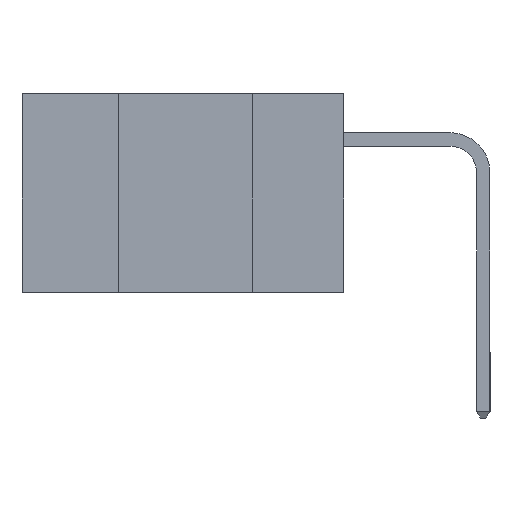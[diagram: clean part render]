
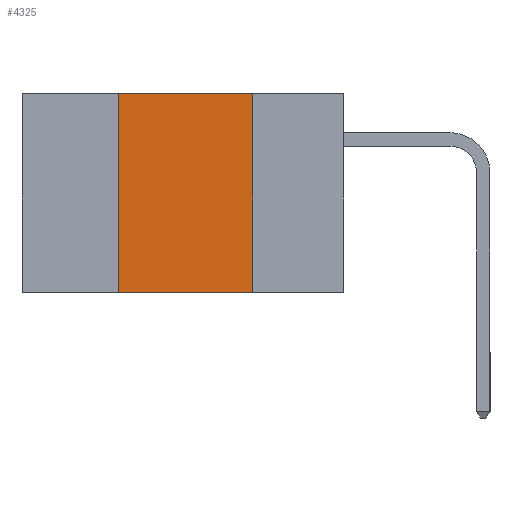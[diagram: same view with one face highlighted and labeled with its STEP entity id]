
A CAD part, left-side view. The second image highlights one B-rep face of the part: STEP entity #4325.
In plain terms, the highlighted planar face has unit normal (-1, 0, 0).
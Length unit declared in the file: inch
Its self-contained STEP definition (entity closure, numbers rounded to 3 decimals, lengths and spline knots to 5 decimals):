
#7 = VERTEX_POINT ( 'NONE', #14242 ) ;
#102 = CARTESIAN_POINT ( 'NONE',  ( 0., 0.42, -0.37 ) ) ;
#1165 = CARTESIAN_POINT ( 'NONE',  ( 0., 0.6, 0. ) ) ;
#1582 = ORIENTED_EDGE ( 'NONE', *, *, #7604, .T. ) ;
#3126 = VECTOR ( 'NONE', #3761, 39.37008 ) ;
#3318 = PLANE ( 'NONE',  #4276 ) ;
#3761 = DIRECTION ( 'NONE',  ( 0., 0., -1. ) ) ;
#4276 = AXIS2_PLACEMENT_3D ( 'NONE', #1165, #6724, #4824 ) ;
#4325 = ADVANCED_FACE ( 'NONE', ( #9241 ), #3318, .F. ) ;
#4824 = DIRECTION ( 'NONE',  ( 0., 0., -1. ) ) ;
#4993 = LINE ( 'NONE', #12678, #24603 ) ;
#4997 = EDGE_CURVE ( 'NONE', #6173, #7, #7768, .T. ) ;
#6173 = VERTEX_POINT ( 'NONE', #9577 ) ;
#6724 = DIRECTION ( 'NONE',  ( 1., 0., 0. ) ) ;
#7172 = VECTOR ( 'NONE', #23172, 39.37008 ) ;
#7604 = EDGE_CURVE ( 'NONE', #20611, #15146, #4993, .T. ) ;
#7768 = LINE ( 'NONE', #23056, #7172 ) ;
#9241 = FACE_OUTER_BOUND ( 'NONE', #16608, .T. ) ;
#9577 = CARTESIAN_POINT ( 'NONE',  ( 0., 0.42, 0. ) ) ;
#10414 = CARTESIAN_POINT ( 'NONE',  ( 0., 0.17, -0.37 ) ) ;
#10953 = CARTESIAN_POINT ( 'NONE',  ( 0., 0.17, -0.37 ) ) ;
#12678 = CARTESIAN_POINT ( 'NONE',  ( 0., 0.6, -0.37 ) ) ;
#13452 = ORIENTED_EDGE ( 'NONE', *, *, #20377, .F. ) ;
#14242 = CARTESIAN_POINT ( 'NONE',  ( 0., 0.17, 0. ) ) ;
#15146 = VERTEX_POINT ( 'NONE', #10414 ) ;
#16549 = CARTESIAN_POINT ( 'NONE',  ( 0., 0.42, -0.37 ) ) ;
#16608 = EDGE_LOOP ( 'NONE', ( #21704, #17305, #13452, #1582 ) ) ;
#16680 = LINE ( 'NONE', #16549, #23276 ) ;
#17148 = LINE ( 'NONE', #10953, #3126 ) ;
#17305 = ORIENTED_EDGE ( 'NONE', *, *, #4997, .F. ) ;
#20377 = EDGE_CURVE ( 'NONE', #20611, #6173, #16680, .T. ) ;
#20423 = DIRECTION ( 'NONE',  ( 0., -1., 0. ) ) ;
#20427 = EDGE_CURVE ( 'NONE', #7, #15146, #17148, .T. ) ;
#20611 = VERTEX_POINT ( 'NONE', #102 ) ;
#21704 = ORIENTED_EDGE ( 'NONE', *, *, #20427, .F. ) ;
#23056 = CARTESIAN_POINT ( 'NONE',  ( 0., 0.6, 0. ) ) ;
#23172 = DIRECTION ( 'NONE',  ( 0., -1., 0. ) ) ;
#23276 = VECTOR ( 'NONE', #24268, 39.37008 ) ;
#24268 = DIRECTION ( 'NONE',  ( 0., 0., 1. ) ) ;
#24603 = VECTOR ( 'NONE', #20423, 39.37008 ) ;
